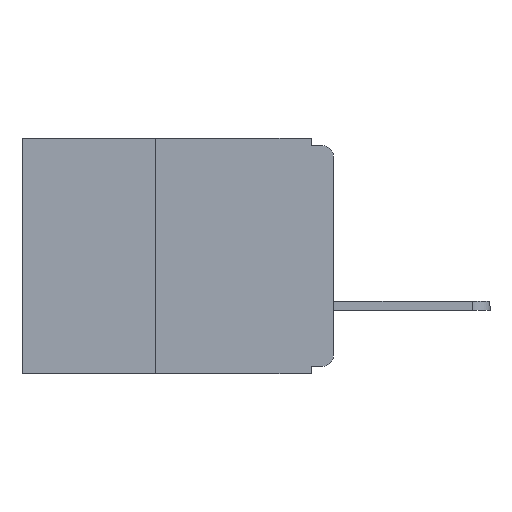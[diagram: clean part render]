
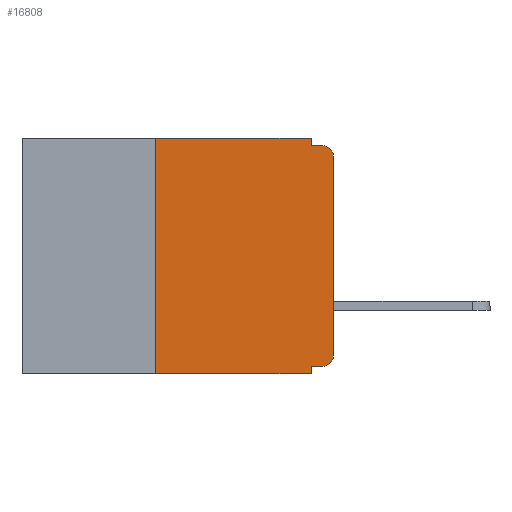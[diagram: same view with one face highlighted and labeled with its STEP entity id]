
A CAD part, left-side view. The second image highlights one B-rep face of the part: STEP entity #16808.
In plain terms, the highlighted planar face has unit normal (-1, 0, 0).
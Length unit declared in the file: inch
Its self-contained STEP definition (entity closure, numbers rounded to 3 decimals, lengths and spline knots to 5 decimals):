
#490 = DIRECTION ( 'NONE',  ( 0., -1., 0. ) ) ;
#568 = PLANE ( 'NONE',  #8473 ) ;
#852 = EDGE_CURVE ( 'NONE', #24883, #21923, #11985, .T. ) ;
#1187 = VERTEX_POINT ( 'NONE', #25085 ) ;
#1474 = ORIENTED_EDGE ( 'NONE', *, *, #9189, .F. ) ;
#2202 = AXIS2_PLACEMENT_3D ( 'NONE', #7340, #20969, #9321 ) ;
#2686 = DIRECTION ( 'NONE',  ( 0., 1., 0. ) ) ;
#3020 = CARTESIAN_POINT ( 'NONE',  ( 0., 0.015, -0.01 ) ) ;
#3060 = ORIENTED_EDGE ( 'NONE', *, *, #23486, .F. ) ;
#3585 = CARTESIAN_POINT ( 'NONE',  ( 0., 0.031, 0. ) ) ;
#4028 = VECTOR ( 'NONE', #7545, 39.37008 ) ;
#4546 = FACE_OUTER_BOUND ( 'NONE', #10679, .T. ) ;
#4819 = VERTEX_POINT ( 'NONE', #21935 ) ;
#4917 = VERTEX_POINT ( 'NONE', #20741 ) ;
#5299 = LINE ( 'NONE', #6192, #22810 ) ;
#6192 = CARTESIAN_POINT ( 'NONE',  ( 0., 0.25, -0.33 ) ) ;
#7340 = CARTESIAN_POINT ( 'NONE',  ( 0., 0.015, -0.305 ) ) ;
#7545 = DIRECTION ( 'NONE',  ( 0., -1., 0. ) ) ;
#7795 = EDGE_CURVE ( 'NONE', #21198, #4917, #22240, .T. ) ;
#8473 = AXIS2_PLACEMENT_3D ( 'NONE', #24243, #14305, #14387 ) ;
#8633 = ORIENTED_EDGE ( 'NONE', *, *, #15057, .T. ) ;
#8739 = EDGE_CURVE ( 'NONE', #24883, #22442, #5299, .T. ) ;
#9189 = EDGE_CURVE ( 'NONE', #22442, #21889, #24951, .T. ) ;
#9321 = DIRECTION ( 'NONE',  ( 0., 0., -1. ) ) ;
#9520 = CARTESIAN_POINT ( 'NONE',  ( 0., 0.437, 0. ) ) ;
#9816 = EDGE_CURVE ( 'NONE', #1187, #20153, #15051, .T. ) ;
#10007 = DIRECTION ( 'NONE',  ( -1., 0., 0. ) ) ;
#10650 = VECTOR ( 'NONE', #490, 39.37008 ) ;
#10655 = CIRCLE ( 'NONE', #2202, 0.015 ) ;
#10679 = EDGE_LOOP ( 'NONE', ( #8633, #12564, #3060, #24618, #1474, #19618, #18710, #16871, #22492, #20928 ) ) ;
#10855 = LINE ( 'NONE', #10903, #19994 ) ;
#10903 = CARTESIAN_POINT ( 'NONE',  ( 0., 0., 0. ) ) ;
#10929 = CARTESIAN_POINT ( 'NONE',  ( 0., 0.015, -0.32 ) ) ;
#11449 = CARTESIAN_POINT ( 'NONE',  ( 0., 0.25, -0.33 ) ) ;
#11519 = DIRECTION ( 'NONE',  ( 0., 0., -1. ) ) ;
#11654 = CARTESIAN_POINT ( 'NONE',  ( 0., 0.031, -0.33 ) ) ;
#11783 = VECTOR ( 'NONE', #2686, 39.37008 ) ;
#11985 = LINE ( 'NONE', #13136, #21823 ) ;
#12564 = ORIENTED_EDGE ( 'NONE', *, *, #9816, .T. ) ;
#12963 = DIRECTION ( 'NONE',  ( 0., -1., 0. ) ) ;
#13086 = CARTESIAN_POINT ( 'NONE',  ( 0., 0.25, 0. ) ) ;
#13136 = CARTESIAN_POINT ( 'NONE',  ( 0., 0.437, -0.33 ) ) ;
#13842 = DIRECTION ( 'NONE',  ( 0., 0., -1. ) ) ;
#14025 = VECTOR ( 'NONE', #13842, 39.37008 ) ;
#14203 = EDGE_CURVE ( 'NONE', #21889, #15552, #21315, .T. ) ;
#14305 = DIRECTION ( 'NONE',  ( 1., 0., 0. ) ) ;
#14387 = DIRECTION ( 'NONE',  ( 0., 0., -1. ) ) ;
#14550 = CARTESIAN_POINT ( 'NONE',  ( 0., 0., -0.32 ) ) ;
#15051 = CIRCLE ( 'NONE', #15058, 0.015 ) ;
#15057 = EDGE_CURVE ( 'NONE', #4819, #1187, #10855, .T. ) ;
#15058 = AXIS2_PLACEMENT_3D ( 'NONE', #21704, #10007, #23732 ) ;
#15447 = VECTOR ( 'NONE', #11519, 39.37008 ) ;
#15552 = VERTEX_POINT ( 'NONE', #24128 ) ;
#15776 = LINE ( 'NONE', #16229, #10650 ) ;
#16229 = CARTESIAN_POINT ( 'NONE',  ( 0., 0., -0.01 ) ) ;
#16808 = ADVANCED_FACE ( 'NONE', ( #4546 ), #568, .F. ) ;
#16871 = ORIENTED_EDGE ( 'NONE', *, *, #22686, .F. ) ;
#17255 = CARTESIAN_POINT ( 'NONE',  ( 0., 0.031, 0. ) ) ;
#18710 = ORIENTED_EDGE ( 'NONE', *, *, #852, .T. ) ;
#19618 = ORIENTED_EDGE ( 'NONE', *, *, #8739, .F. ) ;
#19789 = DIRECTION ( 'NONE',  ( 0., 0., 1. ) ) ;
#19994 = VECTOR ( 'NONE', #20710, 39.37008 ) ;
#20153 = VERTEX_POINT ( 'NONE', #3020 ) ;
#20710 = DIRECTION ( 'NONE',  ( 0., 0., 1. ) ) ;
#20741 = CARTESIAN_POINT ( 'NONE',  ( 0., 0.031, -0.32 ) ) ;
#20928 = ORIENTED_EDGE ( 'NONE', *, *, #24160, .T. ) ;
#20969 = DIRECTION ( 'NONE',  ( -1., 0., 0. ) ) ;
#21198 = VERTEX_POINT ( 'NONE', #10929 ) ;
#21315 = LINE ( 'NONE', #17255, #15447 ) ;
#21704 = CARTESIAN_POINT ( 'NONE',  ( 0., 0.015, -0.025 ) ) ;
#21755 = CARTESIAN_POINT ( 'NONE',  ( 0., 0.031, -0.33 ) ) ;
#21823 = VECTOR ( 'NONE', #12963, 39.37008 ) ;
#21889 = VERTEX_POINT ( 'NONE', #3585 ) ;
#21923 = VERTEX_POINT ( 'NONE', #11654 ) ;
#21935 = CARTESIAN_POINT ( 'NONE',  ( 0., 0., -0.305 ) ) ;
#22240 = LINE ( 'NONE', #14550, #11783 ) ;
#22442 = VERTEX_POINT ( 'NONE', #13086 ) ;
#22492 = ORIENTED_EDGE ( 'NONE', *, *, #7795, .F. ) ;
#22686 = EDGE_CURVE ( 'NONE', #4917, #21923, #24514, .T. ) ;
#22810 = VECTOR ( 'NONE', #19789, 39.37008 ) ;
#23486 = EDGE_CURVE ( 'NONE', #15552, #20153, #15776, .T. ) ;
#23732 = DIRECTION ( 'NONE',  ( 0., 0., -1. ) ) ;
#24128 = CARTESIAN_POINT ( 'NONE',  ( 0., 0.031, -0.01 ) ) ;
#24160 = EDGE_CURVE ( 'NONE', #21198, #4819, #10655, .T. ) ;
#24243 = CARTESIAN_POINT ( 'NONE',  ( 0., 0.437, 0. ) ) ;
#24514 = LINE ( 'NONE', #21755, #14025 ) ;
#24618 = ORIENTED_EDGE ( 'NONE', *, *, #14203, .F. ) ;
#24883 = VERTEX_POINT ( 'NONE', #11449 ) ;
#24951 = LINE ( 'NONE', #9520, #4028 ) ;
#25085 = CARTESIAN_POINT ( 'NONE',  ( 0., 0., -0.025 ) ) ;
